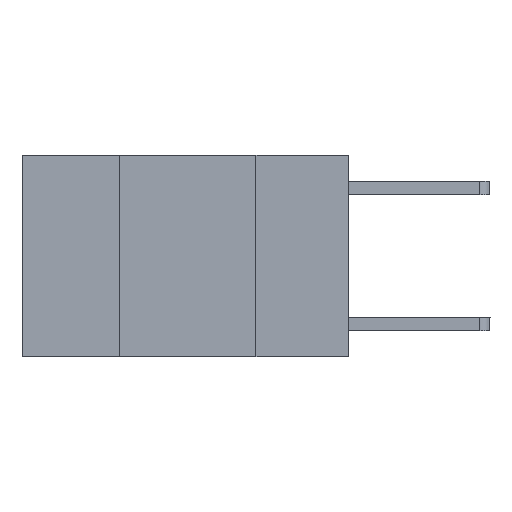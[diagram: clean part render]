
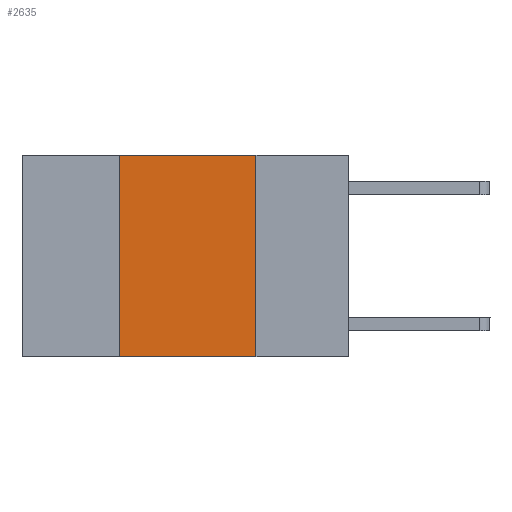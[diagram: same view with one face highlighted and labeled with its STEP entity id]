
A CAD part, left-side view. The second image highlights one B-rep face of the part: STEP entity #2635.
In plain terms, the highlighted planar face has unit normal (-1, 0, 0).
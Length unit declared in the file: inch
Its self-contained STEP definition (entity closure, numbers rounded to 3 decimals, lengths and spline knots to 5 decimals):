
#223 = EDGE_CURVE ( 'NONE', #3684, #10617, #1789, .T. ) ;
#472 = PLANE ( 'NONE',  #10024 ) ;
#678 = EDGE_CURVE ( 'NONE', #10617, #6157, #10200, .T. ) ;
#1167 = DIRECTION ( 'NONE',  ( 0., -1., 0. ) ) ;
#1789 = LINE ( 'NONE', #5145, #6406 ) ;
#2034 = LINE ( 'NONE', #2972, #8918 ) ;
#2080 = ORIENTED_EDGE ( 'NONE', *, *, #7351, .F. ) ;
#2241 = CARTESIAN_POINT ( 'NONE',  ( 0., 0.17, 0. ) ) ;
#2285 = DIRECTION ( 'NONE',  ( 1., 0., 0. ) ) ;
#2635 = ADVANCED_FACE ( 'NONE', ( #4896 ), #472, .F. ) ;
#2788 = ORIENTED_EDGE ( 'NONE', *, *, #678, .F. ) ;
#2802 = EDGE_LOOP ( 'NONE', ( #2080, #2788, #3210, #3949 ) ) ;
#2972 = CARTESIAN_POINT ( 'NONE',  ( 0., 0.6, -0.37 ) ) ;
#3210 = ORIENTED_EDGE ( 'NONE', *, *, #223, .F. ) ;
#3322 = CARTESIAN_POINT ( 'NONE',  ( 0., 0.17, 0. ) ) ;
#3684 = VERTEX_POINT ( 'NONE', #4771 ) ;
#3949 = ORIENTED_EDGE ( 'NONE', *, *, #8324, .T. ) ;
#4425 = VECTOR ( 'NONE', #9928, 39.37008 ) ;
#4771 = CARTESIAN_POINT ( 'NONE',  ( 0., 0.42, -0.37 ) ) ;
#4896 = FACE_OUTER_BOUND ( 'NONE', #2802, .T. ) ;
#4900 = CARTESIAN_POINT ( 'NONE',  ( 0., 0.6, 0. ) ) ;
#5145 = CARTESIAN_POINT ( 'NONE',  ( 0., 0.42, 0. ) ) ;
#6157 = VERTEX_POINT ( 'NONE', #3322 ) ;
#6406 = VECTOR ( 'NONE', #6620, 39.37008 ) ;
#6620 = DIRECTION ( 'NONE',  ( 0., 0., 1. ) ) ;
#6930 = LINE ( 'NONE', #2241, #4425 ) ;
#7007 = VERTEX_POINT ( 'NONE', #7819 ) ;
#7351 = EDGE_CURVE ( 'NONE', #6157, #7007, #6930, .T. ) ;
#7819 = CARTESIAN_POINT ( 'NONE',  ( 0., 0.17, -0.37 ) ) ;
#8324 = EDGE_CURVE ( 'NONE', #3684, #7007, #2034, .T. ) ;
#8330 = DIRECTION ( 'NONE',  ( 0., 0., -1. ) ) ;
#8918 = VECTOR ( 'NONE', #1167, 39.37008 ) ;
#9034 = CARTESIAN_POINT ( 'NONE',  ( 0., 0.42, 0. ) ) ;
#9928 = DIRECTION ( 'NONE',  ( 0., 0., -1. ) ) ;
#9942 = VECTOR ( 'NONE', #10718, 39.37008 ) ;
#10024 = AXIS2_PLACEMENT_3D ( 'NONE', #4900, #2285, #8330 ) ;
#10200 = LINE ( 'NONE', #10863, #9942 ) ;
#10617 = VERTEX_POINT ( 'NONE', #9034 ) ;
#10718 = DIRECTION ( 'NONE',  ( 0., -1., 0. ) ) ;
#10863 = CARTESIAN_POINT ( 'NONE',  ( 0., 0.6, 0. ) ) ;
